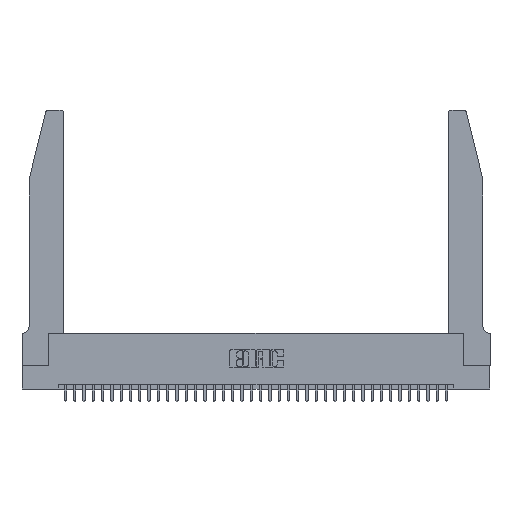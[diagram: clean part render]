
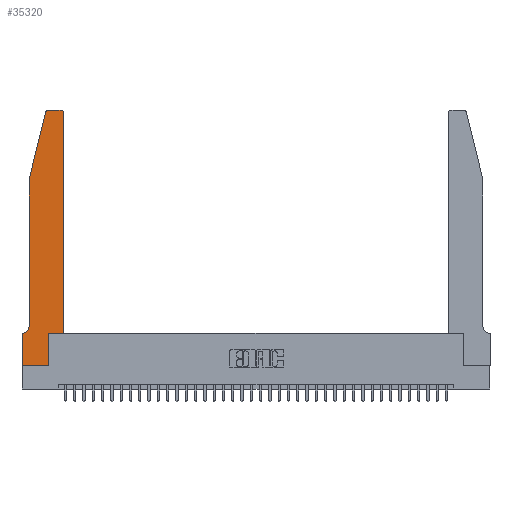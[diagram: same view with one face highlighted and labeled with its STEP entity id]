
A CAD part, top view. The second image highlights one B-rep face of the part: STEP entity #35320.
In plain terms, the highlighted planar face has unit normal (0, 0, 1).
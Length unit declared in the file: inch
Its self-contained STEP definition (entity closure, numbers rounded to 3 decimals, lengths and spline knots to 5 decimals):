
#443 = AXIS2_PLACEMENT_3D ( 'NONE', #1336, #27582, #10251 ) ;
#616 = AXIS2_PLACEMENT_3D ( 'NONE', #17636, #5702, #5389 ) ;
#674 = PLANE ( 'NONE',  #33884 ) ;
#1336 = CARTESIAN_POINT ( 'NONE',  ( 0.0055, 0.42, 0.37 ) ) ;
#1380 = CIRCLE ( 'NONE', #29492, 0.03 ) ;
#1498 = VERTEX_POINT ( 'NONE', #37403 ) ;
#2260 = ORIENTED_EDGE ( 'NONE', *, *, #10927, .T. ) ;
#3095 = CARTESIAN_POINT ( 'NONE',  ( 0.4505, 0.35, 0.37 ) ) ;
#3768 = CARTESIAN_POINT ( 'NONE',  ( 0.2865, 0.35, 0.37 ) ) ;
#3792 = CARTESIAN_POINT ( 'NONE',  ( 0.4205, 2.75, 0.37 ) ) ;
#4068 = VECTOR ( 'NONE', #34537, 39.37008 ) ;
#4498 = VERTEX_POINT ( 'NONE', #22808 ) ;
#4611 = DIRECTION ( 'NONE',  ( -0.239, -0.971, 0. ) ) ;
#5389 = DIRECTION ( 'NONE',  ( 1., 0., 0. ) ) ;
#5702 = DIRECTION ( 'NONE',  ( 0., 0., 1. ) ) ;
#6148 = LINE ( 'NONE', #33207, #27103 ) ;
#6526 = FACE_OUTER_BOUND ( 'NONE', #22634, .T. ) ;
#6781 = ORIENTED_EDGE ( 'NONE', *, *, #17386, .T. ) ;
#7774 = CARTESIAN_POINT ( 'NONE',  ( 0.0755, 2., 0.37 ) ) ;
#7796 = EDGE_CURVE ( 'NONE', #20430, #22609, #21109, .T. ) ;
#7879 = EDGE_CURVE ( 'NONE', #32067, #34213, #8341, .T. ) ;
#8341 = LINE ( 'NONE', #7774, #21575 ) ;
#8521 = CIRCLE ( 'NONE', #616, 0.03 ) ;
#9879 = VERTEX_POINT ( 'NONE', #30298 ) ;
#10251 = DIRECTION ( 'NONE',  ( -1., 0., 0. ) ) ;
#10920 = CARTESIAN_POINT ( 'NONE',  ( 0.2605, 2.75, 0.37 ) ) ;
#10927 = EDGE_CURVE ( 'NONE', #1498, #14937, #27015, .T. ) ;
#11033 = CARTESIAN_POINT ( 'NONE',  ( 0.284, 2.75, 0.37 ) ) ;
#11341 = CARTESIAN_POINT ( 'NONE',  ( 0.4505, 0.35, 0.37 ) ) ;
#11413 = DIRECTION ( 'NONE',  ( 1., 0., 0. ) ) ;
#12399 = DIRECTION ( 'NONE',  ( 0., 0., 1. ) ) ;
#13142 = ORIENTED_EDGE ( 'NONE', *, *, #20488, .T. ) ;
#13354 = CARTESIAN_POINT ( 'NONE',  ( 0.2865, 0.35, 0.37 ) ) ;
#13561 = CARTESIAN_POINT ( 'NONE',  ( 0.0755, 0.35, 0.37 ) ) ;
#14937 = VERTEX_POINT ( 'NONE', #3768 ) ;
#15041 = CARTESIAN_POINT ( 'NONE',  ( 0.4505, 0.35, 0.37 ) ) ;
#15153 = LINE ( 'NONE', #33516, #35240 ) ;
#15641 = ORIENTED_EDGE ( 'NONE', *, *, #19674, .T. ) ;
#16028 = EDGE_CURVE ( 'NONE', #16765, #26585, #8521, .T. ) ;
#16583 = CARTESIAN_POINT ( 'NONE',  ( 0.4505, 2.72, 0.37 ) ) ;
#16765 = VERTEX_POINT ( 'NONE', #16583 ) ;
#16831 = LINE ( 'NONE', #11341, #4068 ) ;
#17386 = EDGE_CURVE ( 'NONE', #26585, #20907, #24740, .T. ) ;
#17509 = ORIENTED_EDGE ( 'NONE', *, *, #7879, .T. ) ;
#17636 = CARTESIAN_POINT ( 'NONE',  ( 0.4205, 2.72, 0.37 ) ) ;
#17655 = CARTESIAN_POINT ( 'NONE',  ( 0.284, 2.72, 0.37 ) ) ;
#17827 = CARTESIAN_POINT ( 'NONE',  ( 0.0755, 0.42, 0.37 ) ) ;
#18398 = CARTESIAN_POINT ( 'NONE',  ( 0., 0.35, 0.37 ) ) ;
#19075 = ORIENTED_EDGE ( 'NONE', *, *, #30271, .T. ) ;
#19448 = ORIENTED_EDGE ( 'NONE', *, *, #30756, .T. ) ;
#19472 = ORIENTED_EDGE ( 'NONE', *, *, #20750, .T. ) ;
#19674 = EDGE_CURVE ( 'NONE', #20907, #32067, #1380, .T. ) ;
#20430 = VERTEX_POINT ( 'NONE', #17827 ) ;
#20488 = EDGE_CURVE ( 'NONE', #22609, #4498, #25000, .T. ) ;
#20666 = ORIENTED_EDGE ( 'NONE', *, *, #37357, .T. ) ;
#20667 = ORIENTED_EDGE ( 'NONE', *, *, #16028, .T. ) ;
#20750 = EDGE_CURVE ( 'NONE', #14937, #37090, #35104, .T. ) ;
#20907 = VERTEX_POINT ( 'NONE', #11033 ) ;
#21048 = DIRECTION ( 'NONE',  ( 1., 0., 0. ) ) ;
#21109 = CIRCLE ( 'NONE', #443, 0.07 ) ;
#21575 = VECTOR ( 'NONE', #4611, 39.37008 ) ;
#22253 = CARTESIAN_POINT ( 'NONE',  ( 0.0755, 2., 0.37 ) ) ;
#22609 = VERTEX_POINT ( 'NONE', #36514 ) ;
#22634 = EDGE_LOOP ( 'NONE', ( #6781, #15641, #17509, #20666, #26251, #13142, #19448, #19075, #2260, #19472, #24106, #20667 ) ) ;
#22808 = CARTESIAN_POINT ( 'NONE',  ( 0., 0.35, 0.37 ) ) ;
#22982 = DIRECTION ( 'NONE',  ( 0., 0., 1. ) ) ;
#23815 = VECTOR ( 'NONE', #34360, 39.37008 ) ;
#24106 = ORIENTED_EDGE ( 'NONE', *, *, #26233, .T. ) ;
#24635 = DIRECTION ( 'NONE',  ( 0., -1., 0. ) ) ;
#24740 = LINE ( 'NONE', #10920, #23815 ) ;
#25000 = LINE ( 'NONE', #13561, #33712 ) ;
#25184 = DIRECTION ( 'NONE',  ( 1., 0., 0. ) ) ;
#25234 = DIRECTION ( 'NONE',  ( -1., 0., 0. ) ) ;
#26233 = EDGE_CURVE ( 'NONE', #37090, #16765, #16831, .T. ) ;
#26251 = ORIENTED_EDGE ( 'NONE', *, *, #7796, .T. ) ;
#26585 = VERTEX_POINT ( 'NONE', #3792 ) ;
#27015 = LINE ( 'NONE', #13354, #30111 ) ;
#27103 = VECTOR ( 'NONE', #36026, 39.37008 ) ;
#27334 = VECTOR ( 'NONE', #29444, 39.37008 ) ;
#27582 = DIRECTION ( 'NONE',  ( 0., 0., -1. ) ) ;
#28766 = LINE ( 'NONE', #33858, #29250 ) ;
#29250 = VECTOR ( 'NONE', #24635, 39.37008 ) ;
#29444 = DIRECTION ( 'NONE',  ( 1., 0., 0. ) ) ;
#29492 = AXIS2_PLACEMENT_3D ( 'NONE', #17655, #22982, #11413 ) ;
#30111 = VECTOR ( 'NONE', #33752, 39.37008 ) ;
#30271 = EDGE_CURVE ( 'NONE', #9879, #1498, #15153, .T. ) ;
#30298 = CARTESIAN_POINT ( 'NONE',  ( 0., 0., 0.37 ) ) ;
#30756 = EDGE_CURVE ( 'NONE', #4498, #9879, #6148, .T. ) ;
#32067 = VERTEX_POINT ( 'NONE', #37553 ) ;
#33207 = CARTESIAN_POINT ( 'NONE',  ( 0., 0., 0.37 ) ) ;
#33516 = CARTESIAN_POINT ( 'NONE',  ( 0., 0., 0.37 ) ) ;
#33712 = VECTOR ( 'NONE', #25234, 39.37008 ) ;
#33752 = DIRECTION ( 'NONE',  ( 0., 1., 0. ) ) ;
#33858 = CARTESIAN_POINT ( 'NONE',  ( 0.0755, 2., 0.37 ) ) ;
#33884 = AXIS2_PLACEMENT_3D ( 'NONE', #18398, #12399, #21048 ) ;
#34213 = VERTEX_POINT ( 'NONE', #22253 ) ;
#34360 = DIRECTION ( 'NONE',  ( -1., 0., 0. ) ) ;
#34537 = DIRECTION ( 'NONE',  ( 0., 1., 0. ) ) ;
#35104 = LINE ( 'NONE', #3095, #27334 ) ;
#35240 = VECTOR ( 'NONE', #25184, 39.37008 ) ;
#35320 = ADVANCED_FACE ( 'NONE', ( #6526 ), #674, .T. ) ;
#36026 = DIRECTION ( 'NONE',  ( 0., -1., 0. ) ) ;
#36514 = CARTESIAN_POINT ( 'NONE',  ( 0.0055, 0.35, 0.37 ) ) ;
#37090 = VERTEX_POINT ( 'NONE', #15041 ) ;
#37357 = EDGE_CURVE ( 'NONE', #34213, #20430, #28766, .T. ) ;
#37403 = CARTESIAN_POINT ( 'NONE',  ( 0.2865, 0., 0.37 ) ) ;
#37553 = CARTESIAN_POINT ( 'NONE',  ( 0.25487, 2.72718, 0.37 ) ) ;
